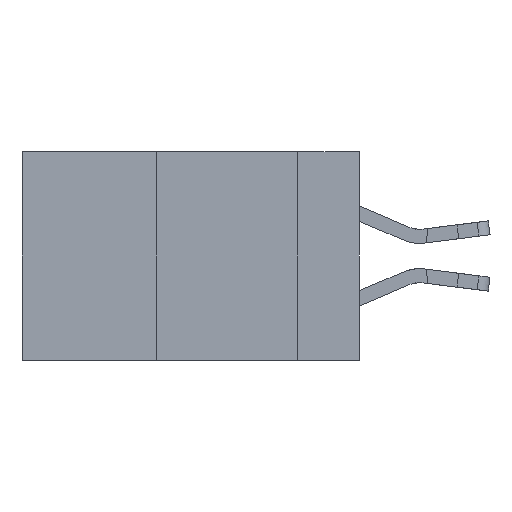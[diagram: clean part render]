
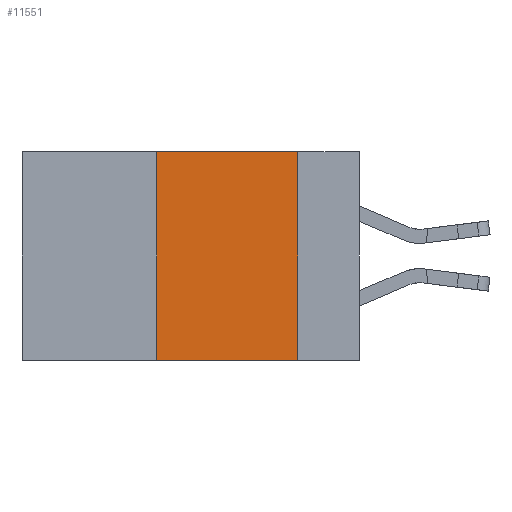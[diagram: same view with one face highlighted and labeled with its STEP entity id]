
A CAD part, left-side view. The second image highlights one B-rep face of the part: STEP entity #11551.
In plain terms, the highlighted planar face has unit normal (-1, 0, 0).
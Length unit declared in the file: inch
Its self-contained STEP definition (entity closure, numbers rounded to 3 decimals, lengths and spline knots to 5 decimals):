
#130 = CARTESIAN_POINT ( 'NONE',  ( 0., 0.36, 0. ) ) ;
#533 = CARTESIAN_POINT ( 'NONE',  ( 0., 0.36, 0. ) ) ;
#2227 = VERTEX_POINT ( 'NONE', #5864 ) ;
#3208 = EDGE_LOOP ( 'NONE', ( #13991, #17424, #8086, #15220 ) ) ;
#3508 = CARTESIAN_POINT ( 'NONE',  ( 0., 0.6, -0.37 ) ) ;
#4116 = LINE ( 'NONE', #10600, #14136 ) ;
#5864 = CARTESIAN_POINT ( 'NONE',  ( 0., 0.11, 0. ) ) ;
#5966 = LINE ( 'NONE', #3508, #6173 ) ;
#6173 = VECTOR ( 'NONE', #13590, 39.37008 ) ;
#7296 = DIRECTION ( 'NONE',  ( 0., 0., -1. ) ) ;
#7776 = FACE_OUTER_BOUND ( 'NONE', #3208, .T. ) ;
#7895 = EDGE_CURVE ( 'NONE', #31008, #2227, #4116, .T. ) ;
#8086 = ORIENTED_EDGE ( 'NONE', *, *, #16547, .F. ) ;
#8475 = CARTESIAN_POINT ( 'NONE',  ( 0., 0.11, -0.37 ) ) ;
#10600 = CARTESIAN_POINT ( 'NONE',  ( 0., 0.6, 0. ) ) ;
#11551 = ADVANCED_FACE ( 'NONE', ( #7776 ), #24917, .F. ) ;
#13051 = CARTESIAN_POINT ( 'NONE',  ( 0., 0.36, -0.37 ) ) ;
#13590 = DIRECTION ( 'NONE',  ( 0., -1., 0. ) ) ;
#13991 = ORIENTED_EDGE ( 'NONE', *, *, #15243, .F. ) ;
#14136 = VECTOR ( 'NONE', #20682, 39.37008 ) ;
#14588 = VERTEX_POINT ( 'NONE', #8475 ) ;
#14862 = DIRECTION ( 'NONE',  ( 0., 0., 1. ) ) ;
#15220 = ORIENTED_EDGE ( 'NONE', *, *, #23712, .T. ) ;
#15243 = EDGE_CURVE ( 'NONE', #2227, #14588, #15620, .T. ) ;
#15351 = VECTOR ( 'NONE', #28097, 39.37008 ) ;
#15620 = LINE ( 'NONE', #20748, #15351 ) ;
#16547 = EDGE_CURVE ( 'NONE', #29669, #31008, #20913, .T. ) ;
#17424 = ORIENTED_EDGE ( 'NONE', *, *, #7895, .F. ) ;
#20682 = DIRECTION ( 'NONE',  ( 0., -1., 0. ) ) ;
#20748 = CARTESIAN_POINT ( 'NONE',  ( 0., 0.11, 0. ) ) ;
#20913 = LINE ( 'NONE', #130, #30085 ) ;
#23323 = AXIS2_PLACEMENT_3D ( 'NONE', #29845, #24767, #7296 ) ;
#23712 = EDGE_CURVE ( 'NONE', #29669, #14588, #5966, .T. ) ;
#24767 = DIRECTION ( 'NONE',  ( 1., 0., 0. ) ) ;
#24917 = PLANE ( 'NONE',  #23323 ) ;
#28097 = DIRECTION ( 'NONE',  ( 0., 0., -1. ) ) ;
#29669 = VERTEX_POINT ( 'NONE', #13051 ) ;
#29845 = CARTESIAN_POINT ( 'NONE',  ( 0., 0.6, 0. ) ) ;
#30085 = VECTOR ( 'NONE', #14862, 39.37008 ) ;
#31008 = VERTEX_POINT ( 'NONE', #533 ) ;
